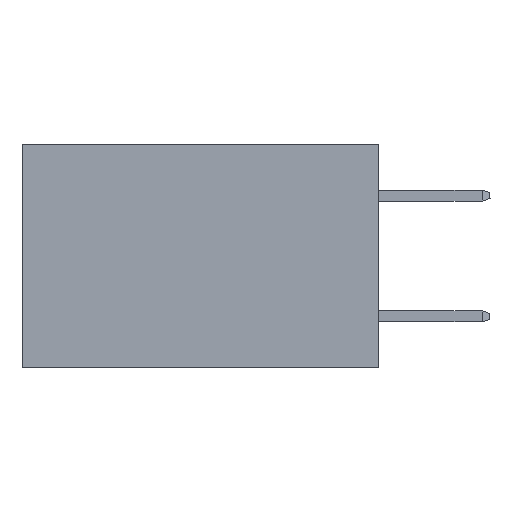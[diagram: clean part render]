
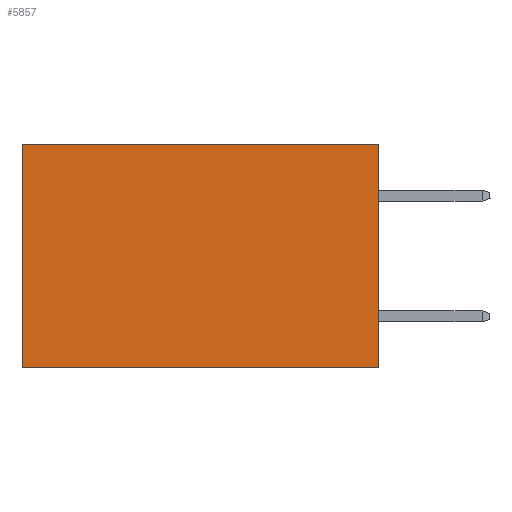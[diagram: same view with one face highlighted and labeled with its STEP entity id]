
A CAD part, left-side view. The second image highlights one B-rep face of the part: STEP entity #5857.
In plain terms, the highlighted planar face has unit normal (-1, 0, 0).
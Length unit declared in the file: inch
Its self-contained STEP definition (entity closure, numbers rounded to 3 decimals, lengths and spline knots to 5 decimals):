
#611 = VECTOR ( 'NONE', #1762, 39.37008 ) ;
#1359 = VERTEX_POINT ( 'NONE', #21275 ) ;
#1371 = LINE ( 'NONE', #5004, #5848 ) ;
#1630 = DIRECTION ( 'NONE',  ( 0., 0., -1. ) ) ;
#1665 = DIRECTION ( 'NONE',  ( 1., 0., 0. ) ) ;
#1698 = CARTESIAN_POINT ( 'NONE',  ( 0.277, 0., -0.37 ) ) ;
#1728 = PLANE ( 'NONE',  #3548 ) ;
#1762 = DIRECTION ( 'NONE',  ( 0., 1., 0. ) ) ;
#1786 = CARTESIAN_POINT ( 'NONE',  ( 0.277, 0., -0.37 ) ) ;
#2356 = VERTEX_POINT ( 'NONE', #10749 ) ;
#3548 = AXIS2_PLACEMENT_3D ( 'NONE', #1698, #1665, #1630 ) ;
#3962 = LINE ( 'NONE', #12160, #22124 ) ;
#4475 = EDGE_CURVE ( 'NONE', #20700, #1359, #3962, .T. ) ;
#5004 = CARTESIAN_POINT ( 'NONE',  ( 0.277, 0., 0. ) ) ;
#5848 = VECTOR ( 'NONE', #18152, 39.37008 ) ;
#5854 = EDGE_CURVE ( 'NONE', #2356, #1359, #18138, .T. ) ;
#5857 = ADVANCED_FACE ( 'NONE', ( #6448 ), #1728, .F. ) ;
#6448 = FACE_OUTER_BOUND ( 'NONE', #26211, .T. ) ;
#7743 = CARTESIAN_POINT ( 'NONE',  ( 0.277, 0., -0.37 ) ) ;
#10658 = LINE ( 'NONE', #7743, #27437 ) ;
#10749 = CARTESIAN_POINT ( 'NONE',  ( 0.277, 0., -0.37 ) ) ;
#11607 = ORIENTED_EDGE ( 'NONE', *, *, #4475, .T. ) ;
#11767 = DIRECTION ( 'NONE',  ( 0., 0., -1. ) ) ;
#12160 = CARTESIAN_POINT ( 'NONE',  ( 0.277, 0.59, -0.37 ) ) ;
#15925 = CARTESIAN_POINT ( 'NONE',  ( 0.277, 0.59, 0. ) ) ;
#18101 = EDGE_CURVE ( 'NONE', #26914, #20700, #1371, .T. ) ;
#18138 = LINE ( 'NONE', #1786, #611 ) ;
#18152 = DIRECTION ( 'NONE',  ( 0., 1., 0. ) ) ;
#20700 = VERTEX_POINT ( 'NONE', #15925 ) ;
#21275 = CARTESIAN_POINT ( 'NONE',  ( 0.277, 0.59, -0.37 ) ) ;
#21481 = ORIENTED_EDGE ( 'NONE', *, *, #18101, .T. ) ;
#22124 = VECTOR ( 'NONE', #11767, 39.37008 ) ;
#23140 = DIRECTION ( 'NONE',  ( 0., 0., -1. ) ) ;
#23772 = ORIENTED_EDGE ( 'NONE', *, *, #5854, .F. ) ;
#24945 = CARTESIAN_POINT ( 'NONE',  ( 0.277, 0., 0. ) ) ;
#25490 = EDGE_CURVE ( 'NONE', #26914, #2356, #10658, .T. ) ;
#26211 = EDGE_LOOP ( 'NONE', ( #11607, #23772, #27761, #21481 ) ) ;
#26914 = VERTEX_POINT ( 'NONE', #24945 ) ;
#27437 = VECTOR ( 'NONE', #23140, 39.37008 ) ;
#27761 = ORIENTED_EDGE ( 'NONE', *, *, #25490, .F. ) ;
